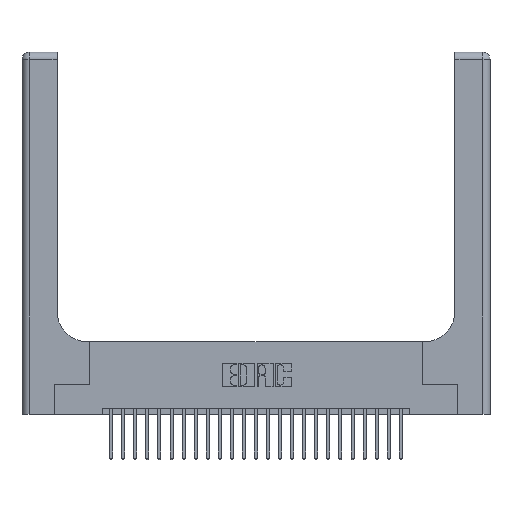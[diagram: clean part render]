
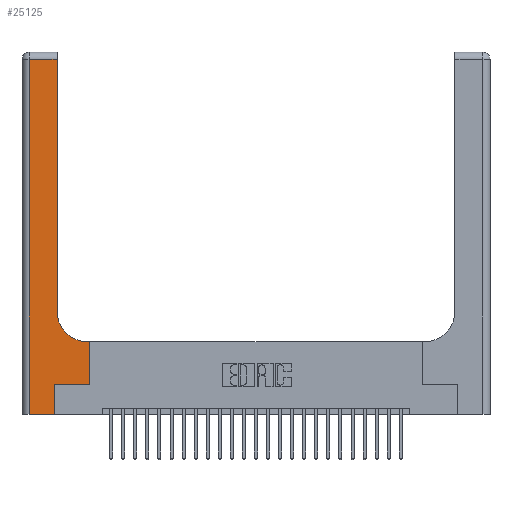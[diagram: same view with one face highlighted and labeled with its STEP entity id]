
A CAD part, top view. The second image highlights one B-rep face of the part: STEP entity #25125.
In plain terms, the highlighted planar face has unit normal (0, 0, 1).
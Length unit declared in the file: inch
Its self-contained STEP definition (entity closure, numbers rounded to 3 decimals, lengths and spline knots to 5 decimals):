
#103 = DIRECTION ( 'NONE',  ( -1., 0., 0. ) ) ;
#217 = VERTEX_POINT ( 'NONE', #7581 ) ;
#719 = LINE ( 'NONE', #20245, #16908 ) ;
#1298 = DIRECTION ( 'NONE',  ( 0., 1., 0. ) ) ;
#1355 = VECTOR ( 'NONE', #24619, 39.37008 ) ;
#1364 = EDGE_CURVE ( 'NONE', #7427, #8073, #19990, .T. ) ;
#1430 = CARTESIAN_POINT ( 'NONE',  ( 0.06, 3., 0.37 ) ) ;
#1859 = CIRCLE ( 'NONE', #17388, 0.25 ) ;
#2028 = LINE ( 'NONE', #22178, #7034 ) ;
#3459 = DIRECTION ( 'NONE',  ( -1., 0., 0. ) ) ;
#3959 = EDGE_CURVE ( 'NONE', #14828, #11608, #5506, .T. ) ;
#4231 = CARTESIAN_POINT ( 'NONE',  ( 0.269, 0.25, 0.37 ) ) ;
#4377 = LINE ( 'NONE', #10198, #21021 ) ;
#5199 = EDGE_CURVE ( 'NONE', #15130, #14828, #719, .T. ) ;
#5506 = LINE ( 'NONE', #16010, #22769 ) ;
#5757 = DIRECTION ( 'NONE',  ( 0., -1., 0. ) ) ;
#6372 = DIRECTION ( 'NONE',  ( 1., 0., 0. ) ) ;
#6795 = CARTESIAN_POINT ( 'NONE',  ( 0.5585, 0.6, 0.37 ) ) ;
#6804 = ORIENTED_EDGE ( 'NONE', *, *, #23361, .T. ) ;
#7034 = VECTOR ( 'NONE', #1298, 39.37008 ) ;
#7123 = EDGE_CURVE ( 'NONE', #27106, #7427, #4377, .T. ) ;
#7427 = VERTEX_POINT ( 'NONE', #15153 ) ;
#7581 = CARTESIAN_POINT ( 'NONE',  ( 0.269, 0.25, 0.37 ) ) ;
#7723 = EDGE_CURVE ( 'NONE', #16195, #27106, #2028, .T. ) ;
#8073 = VERTEX_POINT ( 'NONE', #25394 ) ;
#8266 = LINE ( 'NONE', #24122, #24125 ) ;
#9295 = CARTESIAN_POINT ( 'NONE',  ( 0.2915, 2.94, 0.37 ) ) ;
#10064 = FACE_OUTER_BOUND ( 'NONE', #14409, .T. ) ;
#10190 = DIRECTION ( 'NONE',  ( 0., 0., -1. ) ) ;
#10198 = CARTESIAN_POINT ( 'NONE',  ( 0., 2.94, 0.37 ) ) ;
#10563 = LINE ( 'NONE', #4231, #15394 ) ;
#11608 = VERTEX_POINT ( 'NONE', #22560 ) ;
#12070 = ORIENTED_EDGE ( 'NONE', *, *, #13506, .T. ) ;
#12872 = DIRECTION ( 'NONE',  ( 0., 0., -1. ) ) ;
#13506 = EDGE_CURVE ( 'NONE', #22099, #217, #17483, .T. ) ;
#14409 = EDGE_LOOP ( 'NONE', ( #17814, #23036, #19138, #6804, #12070, #26902, #17262, #24751, #14765 ) ) ;
#14493 = VECTOR ( 'NONE', #5757, 39.37008 ) ;
#14765 = ORIENTED_EDGE ( 'NONE', *, *, #24313, .T. ) ;
#14828 = VERTEX_POINT ( 'NONE', #6795 ) ;
#15130 = VERTEX_POINT ( 'NONE', #22387 ) ;
#15153 = CARTESIAN_POINT ( 'NONE',  ( 0.06, 2.94, 0.37 ) ) ;
#15394 = VECTOR ( 'NONE', #6372, 39.37008 ) ;
#15858 = EDGE_CURVE ( 'NONE', #217, #15130, #10563, .T. ) ;
#16010 = CARTESIAN_POINT ( 'NONE',  ( 0.2915, 0.6, 0.37 ) ) ;
#16195 = VERTEX_POINT ( 'NONE', #19811 ) ;
#16725 = AXIS2_PLACEMENT_3D ( 'NONE', #16841, #12872, #103 ) ;
#16841 = CARTESIAN_POINT ( 'NONE',  ( 0., 3., 0.37 ) ) ;
#16908 = VECTOR ( 'NONE', #24467, 39.37008 ) ;
#17262 = ORIENTED_EDGE ( 'NONE', *, *, #5199, .T. ) ;
#17388 = AXIS2_PLACEMENT_3D ( 'NONE', #22565, #10190, #24628 ) ;
#17483 = LINE ( 'NONE', #20486, #1355 ) ;
#17814 = ORIENTED_EDGE ( 'NONE', *, *, #7723, .T. ) ;
#17992 = DIRECTION ( 'NONE',  ( 1., 0., 0. ) ) ;
#19138 = ORIENTED_EDGE ( 'NONE', *, *, #1364, .T. ) ;
#19811 = CARTESIAN_POINT ( 'NONE',  ( 0.2915, 0.85, 0.37 ) ) ;
#19990 = LINE ( 'NONE', #1430, #14493 ) ;
#20245 = CARTESIAN_POINT ( 'NONE',  ( 0.5585, 0.25, 0.37 ) ) ;
#20486 = CARTESIAN_POINT ( 'NONE',  ( 0.269, 0., 0.37 ) ) ;
#21021 = VECTOR ( 'NONE', #24634, 39.37008 ) ;
#21856 = CARTESIAN_POINT ( 'NONE',  ( 0.269, 0., 0.37 ) ) ;
#22099 = VERTEX_POINT ( 'NONE', #21856 ) ;
#22178 = CARTESIAN_POINT ( 'NONE',  ( 0.2915, 3., 0.37 ) ) ;
#22387 = CARTESIAN_POINT ( 'NONE',  ( 0.5585, 0.25, 0.37 ) ) ;
#22560 = CARTESIAN_POINT ( 'NONE',  ( 0.5415, 0.6, 0.37 ) ) ;
#22565 = CARTESIAN_POINT ( 'NONE',  ( 0.5415, 0.85, 0.37 ) ) ;
#22769 = VECTOR ( 'NONE', #3459, 39.37008 ) ;
#23036 = ORIENTED_EDGE ( 'NONE', *, *, #7123, .T. ) ;
#23361 = EDGE_CURVE ( 'NONE', #8073, #22099, #8266, .T. ) ;
#24122 = CARTESIAN_POINT ( 'NONE',  ( 0., 0., 0.37 ) ) ;
#24125 = VECTOR ( 'NONE', #17992, 39.37008 ) ;
#24313 = EDGE_CURVE ( 'NONE', #11608, #16195, #1859, .T. ) ;
#24467 = DIRECTION ( 'NONE',  ( 0., 1., 0. ) ) ;
#24619 = DIRECTION ( 'NONE',  ( 0., 1., 0. ) ) ;
#24628 = DIRECTION ( 'NONE',  ( 1., 0., 0. ) ) ;
#24634 = DIRECTION ( 'NONE',  ( -1., 0., 0. ) ) ;
#24751 = ORIENTED_EDGE ( 'NONE', *, *, #3959, .T. ) ;
#25125 = ADVANCED_FACE ( 'NONE', ( #10064 ), #25221, .F. ) ;
#25221 = PLANE ( 'NONE',  #16725 ) ;
#25394 = CARTESIAN_POINT ( 'NONE',  ( 0.06, 0., 0.37 ) ) ;
#26902 = ORIENTED_EDGE ( 'NONE', *, *, #15858, .T. ) ;
#27106 = VERTEX_POINT ( 'NONE', #9295 ) ;
